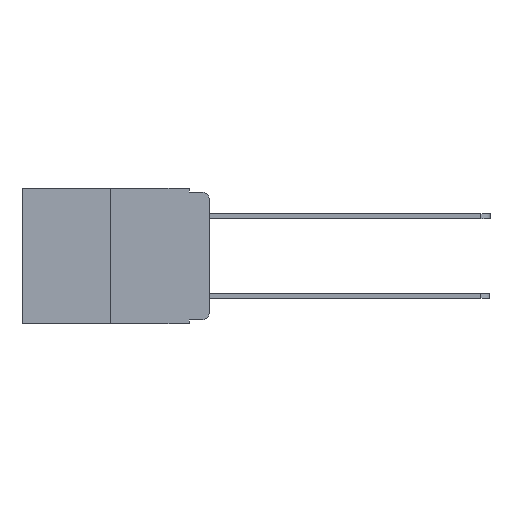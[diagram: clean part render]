
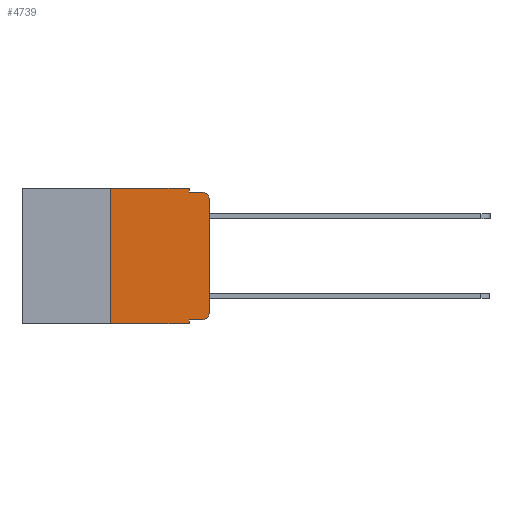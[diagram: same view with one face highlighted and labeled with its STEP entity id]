
A CAD part, left-side view. The second image highlights one B-rep face of the part: STEP entity #4739.
In plain terms, the highlighted planar face has unit normal (-1, 0, 0).
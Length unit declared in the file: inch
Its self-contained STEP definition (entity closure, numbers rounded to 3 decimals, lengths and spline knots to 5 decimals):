
#89 = ORIENTED_EDGE ( 'NONE', *, *, #6262, .T. ) ;
#97 = DIRECTION ( 'NONE',  ( 0., 0., -1. ) ) ;
#400 = CARTESIAN_POINT ( 'NONE',  ( 0., 0.473, 0. ) ) ;
#708 = CARTESIAN_POINT ( 'NONE',  ( 0., 0.051, -0.333 ) ) ;
#768 = CARTESIAN_POINT ( 'NONE',  ( 0., 0., -0.313 ) ) ;
#863 = DIRECTION ( 'NONE',  ( -1., 0., 0. ) ) ;
#1497 = CARTESIAN_POINT ( 'NONE',  ( 0., 0.25, -0.343 ) ) ;
#1506 = LINE ( 'NONE', #708, #9203 ) ;
#1615 = CARTESIAN_POINT ( 'NONE',  ( 0., 0.02, -0.333 ) ) ;
#1671 = EDGE_CURVE ( 'NONE', #5966, #13967, #9005, .T. ) ;
#1680 = CARTESIAN_POINT ( 'NONE',  ( 0., 0.051, 0. ) ) ;
#1730 = CARTESIAN_POINT ( 'NONE',  ( 0., 0.02, -0.01 ) ) ;
#1863 = CARTESIAN_POINT ( 'NONE',  ( 0., 0.051, -0.01 ) ) ;
#2022 = DIRECTION ( 'NONE',  ( 1., 0., 0. ) ) ;
#2269 = CARTESIAN_POINT ( 'NONE',  ( 0., 0.051, -0.01 ) ) ;
#3288 = VECTOR ( 'NONE', #7211, 39.37008 ) ;
#3794 = EDGE_CURVE ( 'NONE', #15718, #13967, #15476, .T. ) ;
#4218 = AXIS2_PLACEMENT_3D ( 'NONE', #400, #2022, #12483 ) ;
#4339 = AXIS2_PLACEMENT_3D ( 'NONE', #13352, #4541, #14841 ) ;
#4500 = VECTOR ( 'NONE', #18730, 39.37008 ) ;
#4541 = DIRECTION ( 'NONE',  ( -1., 0., 0. ) ) ;
#4739 = ADVANCED_FACE ( 'NONE', ( #18314 ), #8154, .F. ) ;
#4839 = EDGE_CURVE ( 'NONE', #9797, #15718, #12654, .T. ) ;
#4901 = CARTESIAN_POINT ( 'NONE',  ( 0., 0.051, 0. ) ) ;
#4954 = CARTESIAN_POINT ( 'NONE',  ( 0., 0.051, -0.343 ) ) ;
#5966 = VERTEX_POINT ( 'NONE', #1863 ) ;
#6262 = EDGE_CURVE ( 'NONE', #7231, #9797, #13969, .T. ) ;
#7211 = DIRECTION ( 'NONE',  ( 0., 0., 1. ) ) ;
#7231 = VERTEX_POINT ( 'NONE', #1615 ) ;
#7258 = VERTEX_POINT ( 'NONE', #1680 ) ;
#7303 = VECTOR ( 'NONE', #16610, 39.37008 ) ;
#8154 = PLANE ( 'NONE',  #4218 ) ;
#8392 = VERTEX_POINT ( 'NONE', #1497 ) ;
#8418 = CARTESIAN_POINT ( 'NONE',  ( 0., 0., 0. ) ) ;
#9005 = LINE ( 'NONE', #2269, #4500 ) ;
#9203 = VECTOR ( 'NONE', #18511, 39.37008 ) ;
#9370 = CARTESIAN_POINT ( 'NONE',  ( 0., 0.051, 0. ) ) ;
#9558 = VERTEX_POINT ( 'NONE', #15276 ) ;
#9603 = VECTOR ( 'NONE', #97, 39.37008 ) ;
#9780 = DIRECTION ( 'NONE',  ( 0., -1., 0. ) ) ;
#9797 = VERTEX_POINT ( 'NONE', #768 ) ;
#9872 = VERTEX_POINT ( 'NONE', #18557 ) ;
#10071 = CARTESIAN_POINT ( 'NONE',  ( 0., 0.02, -0.313 ) ) ;
#10830 = CARTESIAN_POINT ( 'NONE',  ( 0., 0., -0.03 ) ) ;
#11127 = LINE ( 'NONE', #9370, #7303 ) ;
#11128 = EDGE_CURVE ( 'NONE', #9872, #7231, #1506, .T. ) ;
#11423 = DIRECTION ( 'NONE',  ( 0., 0., -1. ) ) ;
#11959 = DIRECTION ( 'NONE',  ( 0., -1., 0. ) ) ;
#11985 = EDGE_CURVE ( 'NONE', #8392, #15742, #17277, .T. ) ;
#12101 = EDGE_CURVE ( 'NONE', #9872, #15742, #11127, .T. ) ;
#12395 = EDGE_LOOP ( 'NONE', ( #13391, #13722, #14411, #14817, #15458, #15480, #15802, #15828, #18902, #89 ) ) ;
#12483 = DIRECTION ( 'NONE',  ( 0., 0., -1. ) ) ;
#12654 = LINE ( 'NONE', #8418, #16112 ) ;
#13352 = CARTESIAN_POINT ( 'NONE',  ( 0., 0.02, -0.03 ) ) ;
#13391 = ORIENTED_EDGE ( 'NONE', *, *, #4839, .T. ) ;
#13722 = ORIENTED_EDGE ( 'NONE', *, *, #3794, .T. ) ;
#13861 = VECTOR ( 'NONE', #11959, 39.37008 ) ;
#13967 = VERTEX_POINT ( 'NONE', #1730 ) ;
#13969 = CIRCLE ( 'NONE', #17511, 0.02 ) ;
#14411 = ORIENTED_EDGE ( 'NONE', *, *, #1671, .F. ) ;
#14817 = ORIENTED_EDGE ( 'NONE', *, *, #17929, .F. ) ;
#14836 = EDGE_CURVE ( 'NONE', #9558, #7258, #15152, .T. ) ;
#14841 = DIRECTION ( 'NONE',  ( 0., 0., -1. ) ) ;
#15152 = LINE ( 'NONE', #16947, #18489 ) ;
#15276 = CARTESIAN_POINT ( 'NONE',  ( 0., 0.25, 0. ) ) ;
#15458 = ORIENTED_EDGE ( 'NONE', *, *, #14836, .F. ) ;
#15476 = CIRCLE ( 'NONE', #4339, 0.02 ) ;
#15480 = ORIENTED_EDGE ( 'NONE', *, *, #16043, .F. ) ;
#15718 = VERTEX_POINT ( 'NONE', #10830 ) ;
#15742 = VERTEX_POINT ( 'NONE', #4954 ) ;
#15802 = ORIENTED_EDGE ( 'NONE', *, *, #11985, .T. ) ;
#15828 = ORIENTED_EDGE ( 'NONE', *, *, #12101, .F. ) ;
#16043 = EDGE_CURVE ( 'NONE', #8392, #9558, #18886, .T. ) ;
#16112 = VECTOR ( 'NONE', #17055, 39.37008 ) ;
#16610 = DIRECTION ( 'NONE',  ( 0., 0., -1. ) ) ;
#16947 = CARTESIAN_POINT ( 'NONE',  ( 0., 0.473, 0. ) ) ;
#17055 = DIRECTION ( 'NONE',  ( 0., 0., 1. ) ) ;
#17277 = LINE ( 'NONE', #19157, #13861 ) ;
#17342 = CARTESIAN_POINT ( 'NONE',  ( 0., 0.25, 0. ) ) ;
#17511 = AXIS2_PLACEMENT_3D ( 'NONE', #10071, #863, #11423 ) ;
#17707 = LINE ( 'NONE', #4901, #9603 ) ;
#17929 = EDGE_CURVE ( 'NONE', #7258, #5966, #17707, .T. ) ;
#18314 = FACE_OUTER_BOUND ( 'NONE', #12395, .T. ) ;
#18489 = VECTOR ( 'NONE', #9780, 39.37008 ) ;
#18511 = DIRECTION ( 'NONE',  ( 0., -1., 0. ) ) ;
#18557 = CARTESIAN_POINT ( 'NONE',  ( 0., 0.051, -0.333 ) ) ;
#18730 = DIRECTION ( 'NONE',  ( 0., -1., 0. ) ) ;
#18886 = LINE ( 'NONE', #17342, #3288 ) ;
#18902 = ORIENTED_EDGE ( 'NONE', *, *, #11128, .T. ) ;
#19157 = CARTESIAN_POINT ( 'NONE',  ( 0., 0.473, -0.343 ) ) ;
